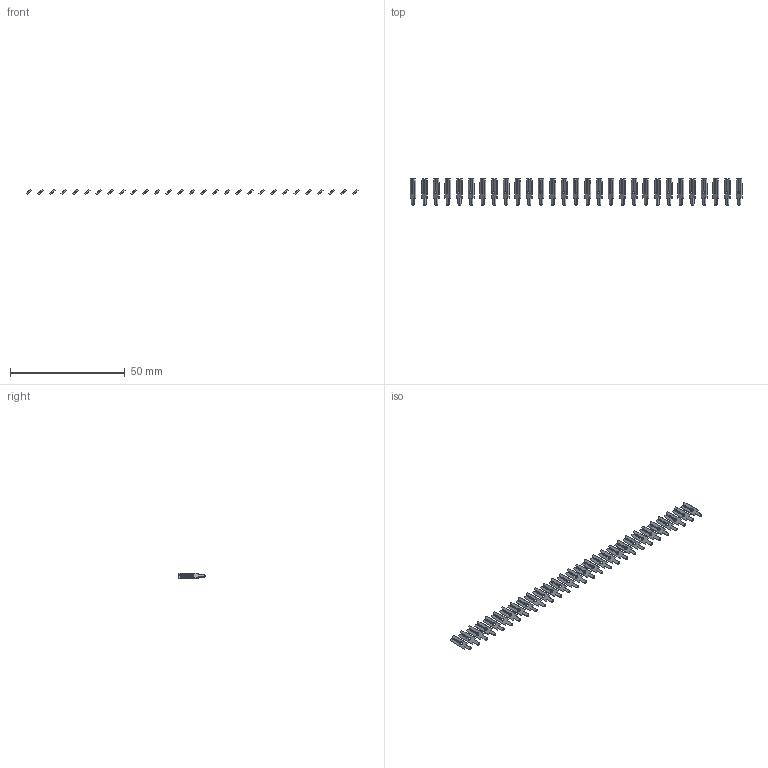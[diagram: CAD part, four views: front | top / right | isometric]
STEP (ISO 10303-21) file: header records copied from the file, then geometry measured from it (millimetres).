
FILE_DESCRIPTION (( 'STEP AP203' ), '1' );
FILE_NAME ('106-029-250-200.STEP', '2020-04-16T19:28:47', ( '' ), ( '' ), 'SwSTEP 2.0', 'SolidWorks 2016', '' );
FILE_SCHEMA (( 'CONFIG_CONTROL_DESIGN' ));
Length unit declared in the file: inch
Products named in the file (2): 106-029-250-200; 100-290-001_100-290-250
Assembly tree (29 placements, depth 2):
  106-029-250-200
    100-290-001_100-290-250  x29
Bounding box: 144.77 x 11.48 x 2.53 mm (x, y, z)
Volume: 452.5 mm3; surface area: 2127.1 mm2
Topology: 29 solids, 29 shells, 696 faces, 1914 edges, 1276 vertices
Faces by surface type: plane 580, cylinder 116
Entity records: 1854 total; most frequent: DIRECTION 182, CARTESIAN_POINT 178, ORIENTED_EDGE 132, DATE_AND_TIME 68, LOCAL_TIME 68, CALENDAR_DATE 68, COORDINATED_UNIVERSAL_TIME_OFFSET 68, EDGE_CURVE 66
